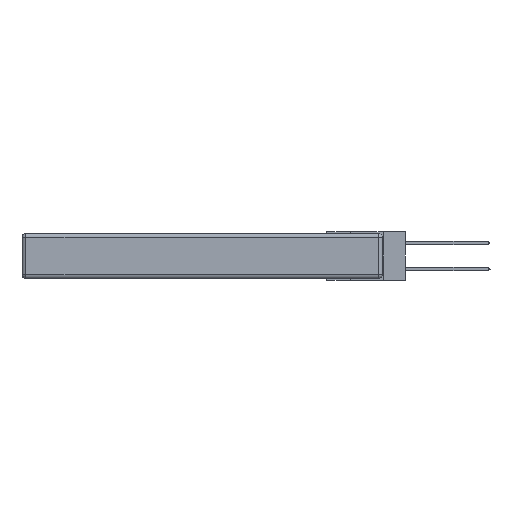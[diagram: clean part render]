
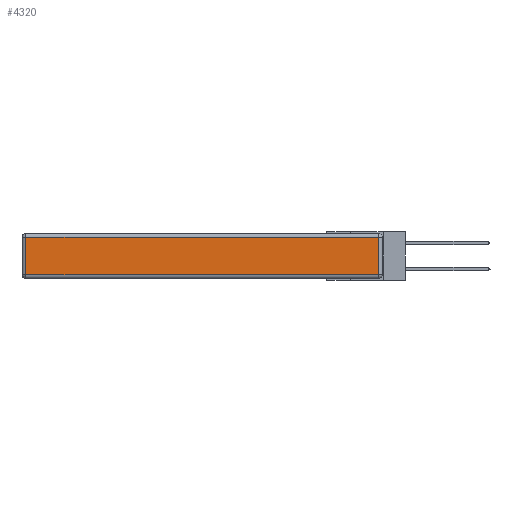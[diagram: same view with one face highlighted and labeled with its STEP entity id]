
A CAD part, left-side view. The second image highlights one B-rep face of the part: STEP entity #4320.
In plain terms, the highlighted planar face has unit normal (-1, 0, 0).
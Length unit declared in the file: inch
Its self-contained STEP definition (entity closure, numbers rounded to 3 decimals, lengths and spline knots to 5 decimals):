
#1930 = EDGE_LOOP ( 'NONE', ( #4792, #11518, #9938, #2542 ) ) ;
#2542 = ORIENTED_EDGE ( 'NONE', *, *, #3911, .T. ) ;
#2952 = EDGE_CURVE ( 'NONE', #14504, #11089, #13832, .T. ) ;
#3911 = EDGE_CURVE ( 'NONE', #13025, #14504, #4476, .T. ) ;
#3996 = VECTOR ( 'NONE', #13088, 39.37008 ) ;
#4292 = VECTOR ( 'NONE', #4480, 39.37008 ) ;
#4320 = ADVANCED_FACE ( 'NONE', ( #6504 ), #11594, .T. ) ;
#4407 = DIRECTION ( 'NONE',  ( -1., 0., 0. ) ) ;
#4476 = LINE ( 'NONE', #15156, #4292 ) ;
#4480 = DIRECTION ( 'NONE',  ( 0., 0., -1. ) ) ;
#4520 = VECTOR ( 'NONE', #9618, 39.37008 ) ;
#4792 = ORIENTED_EDGE ( 'NONE', *, *, #2952, .T. ) ;
#5099 = EDGE_CURVE ( 'NONE', #15141, #13025, #7036, .T. ) ;
#5766 = CARTESIAN_POINT ( 'NONE',  ( 0., 0., -0.343 ) ) ;
#6404 = LINE ( 'NONE', #9273, #3996 ) ;
#6491 = CARTESIAN_POINT ( 'NONE',  ( 0., 0.03, -0.313 ) ) ;
#6504 = FACE_OUTER_BOUND ( 'NONE', #1930, .T. ) ;
#7036 = LINE ( 'NONE', #9405, #11106 ) ;
#8149 = DIRECTION ( 'NONE',  ( 0., 0., 1. ) ) ;
#8310 = CARTESIAN_POINT ( 'NONE',  ( 0., 0., -0.313 ) ) ;
#8586 = DIRECTION ( 'NONE',  ( 0., 1., 0. ) ) ;
#9273 = CARTESIAN_POINT ( 'NONE',  ( 0., 0.03, -0.343 ) ) ;
#9405 = CARTESIAN_POINT ( 'NONE',  ( 0., 2.75, -0.03 ) ) ;
#9618 = DIRECTION ( 'NONE',  ( 0., -1., 0. ) ) ;
#9938 = ORIENTED_EDGE ( 'NONE', *, *, #5099, .T. ) ;
#10874 = AXIS2_PLACEMENT_3D ( 'NONE', #5766, #4407, #8149 ) ;
#11089 = VERTEX_POINT ( 'NONE', #6491 ) ;
#11106 = VECTOR ( 'NONE', #8586, 39.37008 ) ;
#11518 = ORIENTED_EDGE ( 'NONE', *, *, #11924, .T. ) ;
#11527 = CARTESIAN_POINT ( 'NONE',  ( 0., 2.72, -0.313 ) ) ;
#11594 = PLANE ( 'NONE',  #10874 ) ;
#11924 = EDGE_CURVE ( 'NONE', #11089, #15141, #6404, .T. ) ;
#13025 = VERTEX_POINT ( 'NONE', #14145 ) ;
#13088 = DIRECTION ( 'NONE',  ( 0., 0., 1. ) ) ;
#13832 = LINE ( 'NONE', #8310, #4520 ) ;
#14071 = CARTESIAN_POINT ( 'NONE',  ( 0., 0.03, -0.03 ) ) ;
#14145 = CARTESIAN_POINT ( 'NONE',  ( 0., 2.72, -0.03 ) ) ;
#14504 = VERTEX_POINT ( 'NONE', #11527 ) ;
#15141 = VERTEX_POINT ( 'NONE', #14071 ) ;
#15156 = CARTESIAN_POINT ( 'NONE',  ( 0., 2.72, -0.343 ) ) ;
